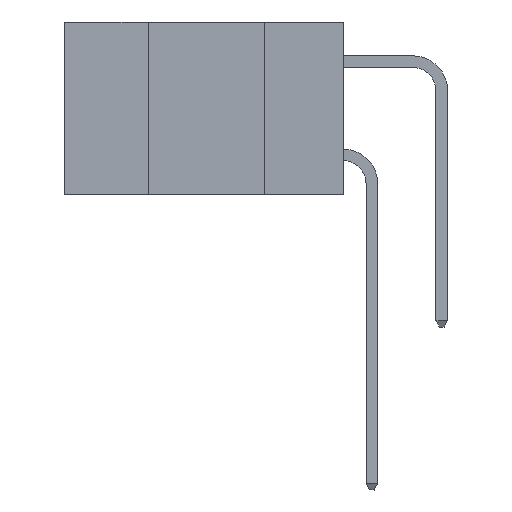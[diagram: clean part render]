
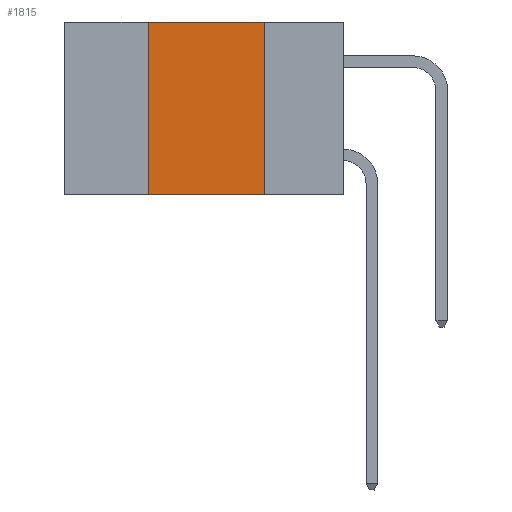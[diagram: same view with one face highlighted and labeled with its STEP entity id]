
A CAD part, left-side view. The second image highlights one B-rep face of the part: STEP entity #1815.
In plain terms, the highlighted planar face has unit normal (-1, 0, 0).
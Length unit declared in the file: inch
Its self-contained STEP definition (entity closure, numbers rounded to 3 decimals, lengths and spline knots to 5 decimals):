
#19 = CARTESIAN_POINT ( 'NONE',  ( 0., 0.42, -0.37 ) ) ;
#39 = CARTESIAN_POINT ( 'NONE',  ( 0., 0.42, -0.37 ) ) ;
#284 = CARTESIAN_POINT ( 'NONE',  ( 0., 0.17, -0.37 ) ) ;
#413 = ORIENTED_EDGE ( 'NONE', *, *, #7665, .T. ) ;
#886 = DIRECTION ( 'NONE',  ( 0., 0., 1. ) ) ;
#1332 = CARTESIAN_POINT ( 'NONE',  ( 0., 0.17, -0.37 ) ) ;
#1507 = VECTOR ( 'NONE', #8250, 39.37008 ) ;
#1795 = EDGE_CURVE ( 'NONE', #3829, #8625, #7912, .T. ) ;
#1815 = ADVANCED_FACE ( 'NONE', ( #3168 ), #6353, .F. ) ;
#2669 = LINE ( 'NONE', #284, #7747 ) ;
#2704 = ORIENTED_EDGE ( 'NONE', *, *, #1795, .F. ) ;
#3168 = FACE_OUTER_BOUND ( 'NONE', #5483, .T. ) ;
#3214 = DIRECTION ( 'NONE',  ( 0., -1., 0. ) ) ;
#3540 = CARTESIAN_POINT ( 'NONE',  ( 0., 0.17, 0. ) ) ;
#3829 = VERTEX_POINT ( 'NONE', #39 ) ;
#4255 = DIRECTION ( 'NONE',  ( 1., 0., 0. ) ) ;
#4781 = VECTOR ( 'NONE', #886, 39.37008 ) ;
#4799 = ORIENTED_EDGE ( 'NONE', *, *, #8115, .F. ) ;
#4998 = VERTEX_POINT ( 'NONE', #1332 ) ;
#5213 = EDGE_CURVE ( 'NONE', #8625, #5352, #7212, .T. ) ;
#5352 = VERTEX_POINT ( 'NONE', #3540 ) ;
#5483 = EDGE_LOOP ( 'NONE', ( #4799, #8415, #2704, #413 ) ) ;
#5898 = CARTESIAN_POINT ( 'NONE',  ( 0., 0.6, -0.37 ) ) ;
#5968 = CARTESIAN_POINT ( 'NONE',  ( 0., 0.42, 0. ) ) ;
#6353 = PLANE ( 'NONE',  #6973 ) ;
#6630 = DIRECTION ( 'NONE',  ( 0., 0., -1. ) ) ;
#6631 = DIRECTION ( 'NONE',  ( 0., 0., -1. ) ) ;
#6973 = AXIS2_PLACEMENT_3D ( 'NONE', #9065, #4255, #6631 ) ;
#7212 = LINE ( 'NONE', #10396, #7856 ) ;
#7665 = EDGE_CURVE ( 'NONE', #3829, #4998, #8790, .T. ) ;
#7747 = VECTOR ( 'NONE', #6630, 39.37008 ) ;
#7856 = VECTOR ( 'NONE', #3214, 39.37008 ) ;
#7912 = LINE ( 'NONE', #19, #4781 ) ;
#8115 = EDGE_CURVE ( 'NONE', #5352, #4998, #2669, .T. ) ;
#8250 = DIRECTION ( 'NONE',  ( 0., -1., 0. ) ) ;
#8415 = ORIENTED_EDGE ( 'NONE', *, *, #5213, .F. ) ;
#8625 = VERTEX_POINT ( 'NONE', #5968 ) ;
#8790 = LINE ( 'NONE', #5898, #1507 ) ;
#9065 = CARTESIAN_POINT ( 'NONE',  ( 0., 0.6, 0. ) ) ;
#10396 = CARTESIAN_POINT ( 'NONE',  ( 0., 0.6, 0. ) ) ;
